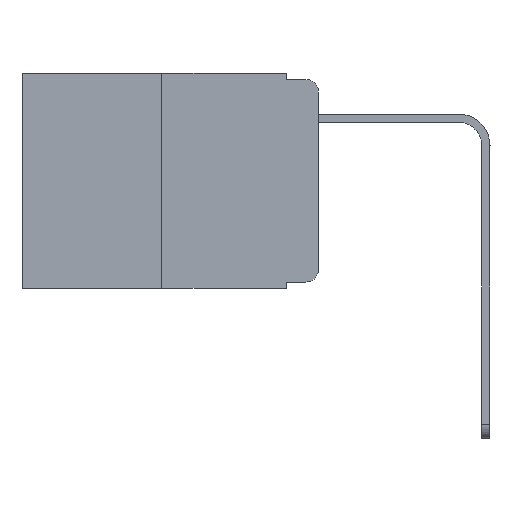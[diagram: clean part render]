
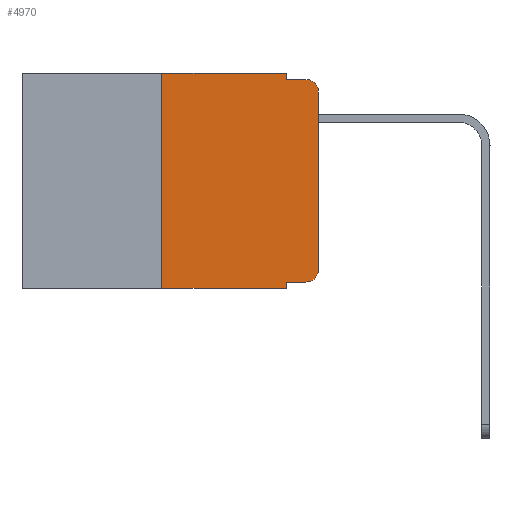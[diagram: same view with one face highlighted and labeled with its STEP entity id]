
A CAD part, left-side view. The second image highlights one B-rep face of the part: STEP entity #4970.
In plain terms, the highlighted planar face has unit normal (-1, 0, 0).
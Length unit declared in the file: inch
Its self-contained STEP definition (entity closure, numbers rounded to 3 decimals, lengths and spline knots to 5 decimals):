
#68 = VECTOR ( 'NONE', #5982, 39.37008 ) ;
#191 = VERTEX_POINT ( 'NONE', #8810 ) ;
#248 = LINE ( 'NONE', #6166, #68 ) ;
#282 = CARTESIAN_POINT ( 'NONE',  ( 0., 0.051, -0.343 ) ) ;
#338 = EDGE_CURVE ( 'NONE', #484, #3695, #248, .T. ) ;
#348 = CARTESIAN_POINT ( 'NONE',  ( 0., 0.02, -0.313 ) ) ;
#389 = ORIENTED_EDGE ( 'NONE', *, *, #12834, .T. ) ;
#484 = VERTEX_POINT ( 'NONE', #4229 ) ;
#586 = DIRECTION ( 'NONE',  ( -1., 0., 0. ) ) ;
#676 = AXIS2_PLACEMENT_3D ( 'NONE', #348, #11937, #5506 ) ;
#1067 = LINE ( 'NONE', #12457, #12582 ) ;
#1088 = DIRECTION ( 'NONE',  ( 0., -1., 0. ) ) ;
#2001 = LINE ( 'NONE', #5933, #8687 ) ;
#2094 = CARTESIAN_POINT ( 'NONE',  ( 0., 0.473, -0.343 ) ) ;
#2120 = EDGE_CURVE ( 'NONE', #7652, #8526, #8355, .T. ) ;
#2149 = EDGE_CURVE ( 'NONE', #3695, #8526, #2001, .T. ) ;
#2392 = FACE_OUTER_BOUND ( 'NONE', #10076, .T. ) ;
#2612 = EDGE_CURVE ( 'NONE', #191, #13266, #3463, .T. ) ;
#2619 = VECTOR ( 'NONE', #5013, 39.37008 ) ;
#2988 = AXIS2_PLACEMENT_3D ( 'NONE', #6959, #586, #8046 ) ;
#3197 = AXIS2_PLACEMENT_3D ( 'NONE', #7315, #8394, #9465 ) ;
#3304 = EDGE_CURVE ( 'NONE', #11461, #6341, #6777, .T. ) ;
#3337 = ORIENTED_EDGE ( 'NONE', *, *, #2612, .T. ) ;
#3463 = LINE ( 'NONE', #3934, #2619 ) ;
#3695 = VERTEX_POINT ( 'NONE', #6887 ) ;
#3746 = DIRECTION ( 'NONE',  ( 0., -1., 0. ) ) ;
#3934 = CARTESIAN_POINT ( 'NONE',  ( 0., 0.051, -0.333 ) ) ;
#4229 = CARTESIAN_POINT ( 'NONE',  ( 0., 0.051, 0. ) ) ;
#4730 = ORIENTED_EDGE ( 'NONE', *, *, #3304, .F. ) ;
#4956 = CIRCLE ( 'NONE', #676, 0.02 ) ;
#4964 = DIRECTION ( 'NONE',  ( 0., -1., 0. ) ) ;
#4970 = ADVANCED_FACE ( 'NONE', ( #2392 ), #12657, .F. ) ;
#5013 = DIRECTION ( 'NONE',  ( 0., -1., 0. ) ) ;
#5486 = CARTESIAN_POINT ( 'NONE',  ( 0., 0.051, 0. ) ) ;
#5506 = DIRECTION ( 'NONE',  ( 0., 0., -1. ) ) ;
#5933 = CARTESIAN_POINT ( 'NONE',  ( 0., 0.051, -0.01 ) ) ;
#5982 = DIRECTION ( 'NONE',  ( 0., 0., -1. ) ) ;
#6166 = CARTESIAN_POINT ( 'NONE',  ( 0., 0.051, 0. ) ) ;
#6327 = LINE ( 'NONE', #11591, #12359 ) ;
#6341 = VERTEX_POINT ( 'NONE', #8086 ) ;
#6373 = CARTESIAN_POINT ( 'NONE',  ( 0., 0.25, 0. ) ) ;
#6404 = VECTOR ( 'NONE', #11786, 39.37008 ) ;
#6777 = LINE ( 'NONE', #6373, #10647 ) ;
#6887 = CARTESIAN_POINT ( 'NONE',  ( 0., 0.051, -0.01 ) ) ;
#6959 = CARTESIAN_POINT ( 'NONE',  ( 0., 0.02, -0.03 ) ) ;
#7315 = CARTESIAN_POINT ( 'NONE',  ( 0., 0.473, 0. ) ) ;
#7499 = CARTESIAN_POINT ( 'NONE',  ( 0., 0., -0.03 ) ) ;
#7607 = ORIENTED_EDGE ( 'NONE', *, *, #2120, .T. ) ;
#7652 = VERTEX_POINT ( 'NONE', #7499 ) ;
#7714 = VERTEX_POINT ( 'NONE', #9845 ) ;
#8024 = ORIENTED_EDGE ( 'NONE', *, *, #9862, .F. ) ;
#8046 = DIRECTION ( 'NONE',  ( 0., 0., -1. ) ) ;
#8086 = CARTESIAN_POINT ( 'NONE',  ( 0., 0.25, 0. ) ) ;
#8180 = ORIENTED_EDGE ( 'NONE', *, *, #10822, .F. ) ;
#8355 = CIRCLE ( 'NONE', #2988, 0.02 ) ;
#8394 = DIRECTION ( 'NONE',  ( 1., 0., 0. ) ) ;
#8526 = VERTEX_POINT ( 'NONE', #13176 ) ;
#8687 = VECTOR ( 'NONE', #4964, 39.37008 ) ;
#8810 = CARTESIAN_POINT ( 'NONE',  ( 0., 0.051, -0.333 ) ) ;
#9163 = CARTESIAN_POINT ( 'NONE',  ( 0., 0.02, -0.333 ) ) ;
#9187 = CARTESIAN_POINT ( 'NONE',  ( 0., 0.25, -0.343 ) ) ;
#9465 = DIRECTION ( 'NONE',  ( 0., 0., -1. ) ) ;
#9845 = CARTESIAN_POINT ( 'NONE',  ( 0., 0., -0.313 ) ) ;
#9862 = EDGE_CURVE ( 'NONE', #191, #12370, #13762, .T. ) ;
#10076 = EDGE_LOOP ( 'NONE', ( #13651, #7607, #11820, #12564, #8180, #4730, #389, #8024, #3337, #10758 ) ) ;
#10647 = VECTOR ( 'NONE', #12879, 39.37008 ) ;
#10758 = ORIENTED_EDGE ( 'NONE', *, *, #13610, .T. ) ;
#10822 = EDGE_CURVE ( 'NONE', #6341, #484, #1067, .T. ) ;
#11461 = VERTEX_POINT ( 'NONE', #9187 ) ;
#11591 = CARTESIAN_POINT ( 'NONE',  ( 0., 0., 0. ) ) ;
#11723 = DIRECTION ( 'NONE',  ( 0., 0., 1. ) ) ;
#11786 = DIRECTION ( 'NONE',  ( 0., 0., -1. ) ) ;
#11820 = ORIENTED_EDGE ( 'NONE', *, *, #2149, .F. ) ;
#11937 = DIRECTION ( 'NONE',  ( -1., 0., 0. ) ) ;
#12078 = EDGE_CURVE ( 'NONE', #7714, #7652, #6327, .T. ) ;
#12330 = VECTOR ( 'NONE', #1088, 39.37008 ) ;
#12359 = VECTOR ( 'NONE', #11723, 39.37008 ) ;
#12370 = VERTEX_POINT ( 'NONE', #282 ) ;
#12457 = CARTESIAN_POINT ( 'NONE',  ( 0., 0.473, 0. ) ) ;
#12564 = ORIENTED_EDGE ( 'NONE', *, *, #338, .F. ) ;
#12582 = VECTOR ( 'NONE', #3746, 39.37008 ) ;
#12657 = PLANE ( 'NONE',  #3197 ) ;
#12834 = EDGE_CURVE ( 'NONE', #11461, #12370, #13662, .T. ) ;
#12879 = DIRECTION ( 'NONE',  ( 0., 0., 1. ) ) ;
#13176 = CARTESIAN_POINT ( 'NONE',  ( 0., 0.02, -0.01 ) ) ;
#13266 = VERTEX_POINT ( 'NONE', #9163 ) ;
#13610 = EDGE_CURVE ( 'NONE', #13266, #7714, #4956, .T. ) ;
#13651 = ORIENTED_EDGE ( 'NONE', *, *, #12078, .T. ) ;
#13662 = LINE ( 'NONE', #2094, #12330 ) ;
#13762 = LINE ( 'NONE', #5486, #6404 ) ;
